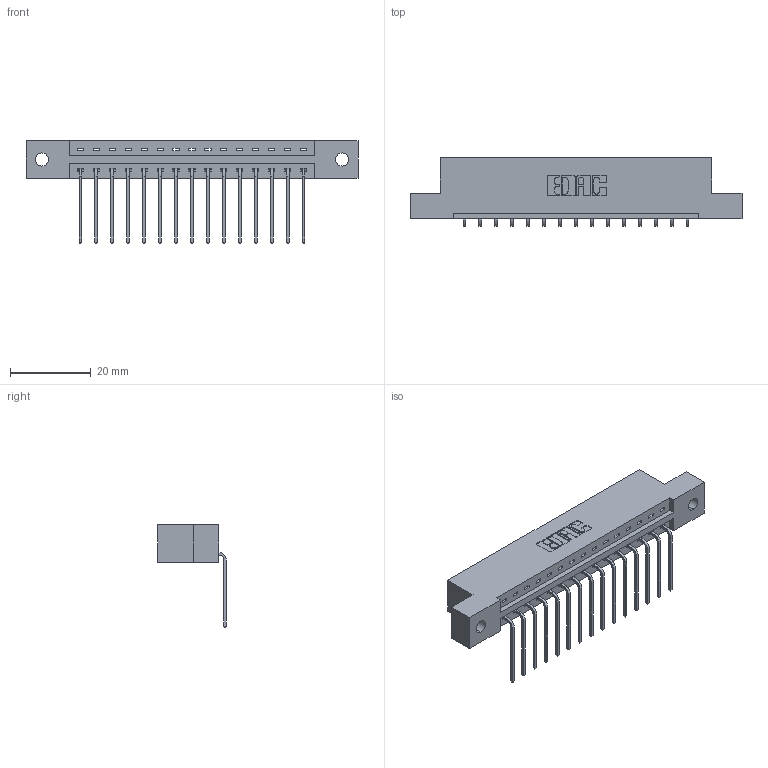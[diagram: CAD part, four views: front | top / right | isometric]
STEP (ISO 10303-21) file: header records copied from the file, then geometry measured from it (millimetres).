
FILE_DESCRIPTION (( 'STEP AP203' ), '1' );
FILE_NAME ('387-015-559-102.STEP', '2019-10-02T17:50:18', ( '' ), ( '' ), 'SwSTEP 2.0', 'SolidWorks 2016', '' );
FILE_SCHEMA (( 'CONFIG_CONTROL_DESIGN' ));
Length unit declared in the file: inch
Products named in the file (3): 337 Part_Flush Mounting Lugs - 0.128 Dia; 387-015-559-102; 345-292-001_558 559 Tail - 1
Assembly tree (16 placements, depth 2):
  387-015-559-102
    337 Part_Flush Mounting Lugs - 0.128 Dia
    345-292-001_558 559 Tail - 1  x15
Bounding box: 82.45 x 17.09 x 25.53 mm (x, y, z)
Volume: 8244.5 mm3; surface area: 8406.8 mm2
Topology: 16 solids, 16 shells, 1074 faces, 3221 edges, 2126 vertices
Faces by surface type: plane 790, cylinder 284
Entity records: 14729 total; most frequent: CARTESIAN_POINT 2571, ORIENTED_EDGE 2522, DIRECTION 2219, EDGE_CURVE 1261, VECTOR 1133, LINE 1133, VERTEX_POINT 838, AXIS2_PLACEMENT_3D 543
